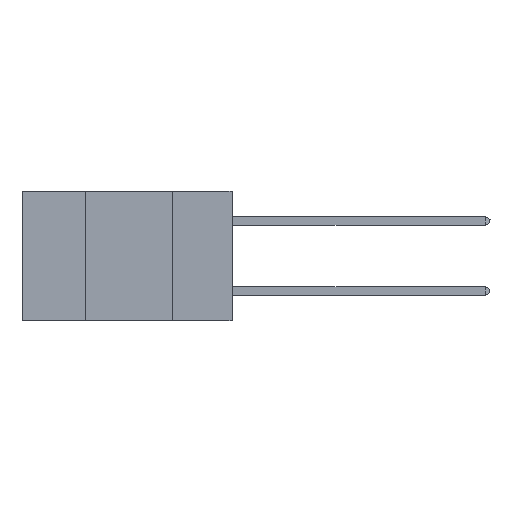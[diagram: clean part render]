
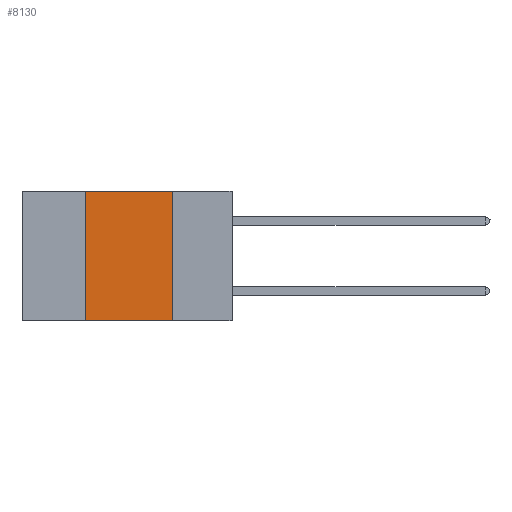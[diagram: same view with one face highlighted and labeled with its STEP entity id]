
A CAD part, left-side view. The second image highlights one B-rep face of the part: STEP entity #8130.
In plain terms, the highlighted planar face has unit normal (-1, 0, 0).
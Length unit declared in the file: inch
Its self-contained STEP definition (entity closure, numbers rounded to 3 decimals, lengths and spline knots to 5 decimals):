
#310 = DIRECTION ( 'NONE',  ( 1., 0., 0. ) ) ;
#503 = EDGE_CURVE ( 'NONE', #17709, #25466, #10288, .T. ) ;
#517 = VERTEX_POINT ( 'NONE', #13190 ) ;
#524 = DIRECTION ( 'NONE',  ( 0., 0., -1. ) ) ;
#1549 = EDGE_CURVE ( 'NONE', #9387, #517, #17278, .T. ) ;
#3550 = CARTESIAN_POINT ( 'NONE',  ( 0., 0.6, 0. ) ) ;
#3720 = LINE ( 'NONE', #23566, #27807 ) ;
#6125 = ORIENTED_EDGE ( 'NONE', *, *, #1549, .T. ) ;
#7242 = LINE ( 'NONE', #11984, #21804 ) ;
#7705 = FACE_OUTER_BOUND ( 'NONE', #16447, .T. ) ;
#8130 = ADVANCED_FACE ( 'NONE', ( #7705 ), #14981, .F. ) ;
#8197 = CARTESIAN_POINT ( 'NONE',  ( 0., 0.6, -0.37 ) ) ;
#8248 = ORIENTED_EDGE ( 'NONE', *, *, #24070, .F. ) ;
#9387 = VERTEX_POINT ( 'NONE', #27971 ) ;
#10288 = LINE ( 'NONE', #3550, #16786 ) ;
#11984 = CARTESIAN_POINT ( 'NONE',  ( 0., 0.42, 0. ) ) ;
#13190 = CARTESIAN_POINT ( 'NONE',  ( 0., 0.17, -0.37 ) ) ;
#14981 = PLANE ( 'NONE',  #20526 ) ;
#16447 = EDGE_LOOP ( 'NONE', ( #8248, #24132, #30494, #6125 ) ) ;
#16786 = VECTOR ( 'NONE', #18222, 39.37008 ) ;
#17278 = LINE ( 'NONE', #8197, #27165 ) ;
#17709 = VERTEX_POINT ( 'NONE', #26209 ) ;
#18222 = DIRECTION ( 'NONE',  ( 0., -1., 0. ) ) ;
#20089 = CARTESIAN_POINT ( 'NONE',  ( 0., 0.6, 0. ) ) ;
#20526 = AXIS2_PLACEMENT_3D ( 'NONE', #20089, #310, #524 ) ;
#21804 = VECTOR ( 'NONE', #21846, 39.37008 ) ;
#21846 = DIRECTION ( 'NONE',  ( 0., 0., 1. ) ) ;
#23566 = CARTESIAN_POINT ( 'NONE',  ( 0., 0.17, 0. ) ) ;
#24070 = EDGE_CURVE ( 'NONE', #25466, #517, #3720, .T. ) ;
#24132 = ORIENTED_EDGE ( 'NONE', *, *, #503, .F. ) ;
#25466 = VERTEX_POINT ( 'NONE', #25894 ) ;
#25894 = CARTESIAN_POINT ( 'NONE',  ( 0., 0.17, 0. ) ) ;
#26209 = CARTESIAN_POINT ( 'NONE',  ( 0., 0.42, 0. ) ) ;
#26504 = DIRECTION ( 'NONE',  ( 0., 0., -1. ) ) ;
#27165 = VECTOR ( 'NONE', #27399, 39.37008 ) ;
#27399 = DIRECTION ( 'NONE',  ( 0., -1., 0. ) ) ;
#27807 = VECTOR ( 'NONE', #26504, 39.37008 ) ;
#27971 = CARTESIAN_POINT ( 'NONE',  ( 0., 0.42, -0.37 ) ) ;
#28797 = EDGE_CURVE ( 'NONE', #9387, #17709, #7242, .T. ) ;
#30494 = ORIENTED_EDGE ( 'NONE', *, *, #28797, .F. ) ;
